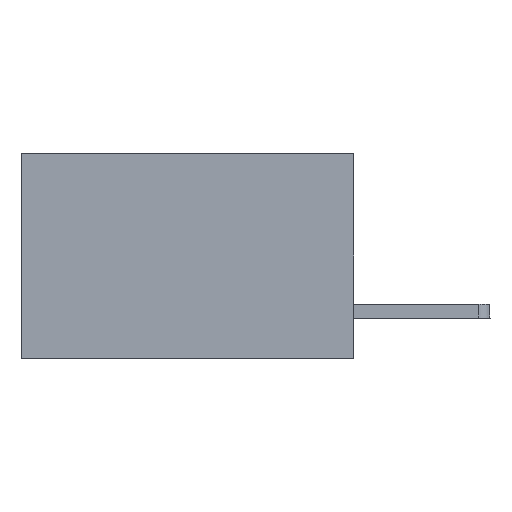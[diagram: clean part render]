
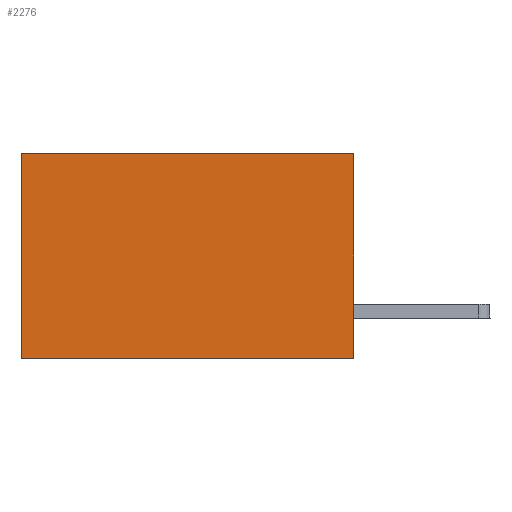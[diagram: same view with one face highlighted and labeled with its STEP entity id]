
A CAD part, left-side view. The second image highlights one B-rep face of the part: STEP entity #2276.
In plain terms, the highlighted planar face has unit normal (-1, 0, 0).
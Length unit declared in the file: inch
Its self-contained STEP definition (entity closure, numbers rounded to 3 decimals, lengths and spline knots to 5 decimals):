
#83 = LINE ( 'NONE', #14897, #2909 ) ;
#582 = EDGE_LOOP ( 'NONE', ( #8738, #12681, #991, #12155 ) ) ;
#651 = VERTEX_POINT ( 'NONE', #6128 ) ;
#991 = ORIENTED_EDGE ( 'NONE', *, *, #5662, .F. ) ;
#1523 = LINE ( 'NONE', #3004, #14735 ) ;
#2205 = DIRECTION ( 'NONE',  ( 0., 0., -1. ) ) ;
#2276 = ADVANCED_FACE ( 'NONE', ( #2409 ), #13121, .F. ) ;
#2409 = FACE_OUTER_BOUND ( 'NONE', #582, .T. ) ;
#2530 = DIRECTION ( 'NONE',  ( 0., 1., 0. ) ) ;
#2909 = VECTOR ( 'NONE', #5752, 39.37008 ) ;
#3004 = CARTESIAN_POINT ( 'NONE',  ( 0.2875, 0., -0.37 ) ) ;
#3277 = EDGE_CURVE ( 'NONE', #11011, #12701, #1523, .T. ) ;
#3392 = CARTESIAN_POINT ( 'NONE',  ( 0.2875, 0., -0.37 ) ) ;
#3790 = VECTOR ( 'NONE', #7036, 39.37008 ) ;
#4533 = EDGE_CURVE ( 'NONE', #651, #12701, #9919, .T. ) ;
#5180 = AXIS2_PLACEMENT_3D ( 'NONE', #12058, #12765, #2205 ) ;
#5662 = EDGE_CURVE ( 'NONE', #13870, #11011, #7246, .T. ) ;
#5752 = DIRECTION ( 'NONE',  ( 0., 1., 0. ) ) ;
#6128 = CARTESIAN_POINT ( 'NONE',  ( 0.2875, 0.6, 0. ) ) ;
#7036 = DIRECTION ( 'NONE',  ( 0., 0., -1. ) ) ;
#7246 = LINE ( 'NONE', #10800, #3790 ) ;
#8738 = ORIENTED_EDGE ( 'NONE', *, *, #4533, .T. ) ;
#9917 = DIRECTION ( 'NONE',  ( 0., 0., -1. ) ) ;
#9919 = LINE ( 'NONE', #12783, #16495 ) ;
#10268 = EDGE_CURVE ( 'NONE', #13870, #651, #83, .T. ) ;
#10800 = CARTESIAN_POINT ( 'NONE',  ( 0.2875, 0., 0. ) ) ;
#10959 = CARTESIAN_POINT ( 'NONE',  ( 0.2875, 0., 0. ) ) ;
#11011 = VERTEX_POINT ( 'NONE', #3392 ) ;
#12058 = CARTESIAN_POINT ( 'NONE',  ( 0.2875, 0., 0. ) ) ;
#12155 = ORIENTED_EDGE ( 'NONE', *, *, #10268, .T. ) ;
#12681 = ORIENTED_EDGE ( 'NONE', *, *, #3277, .F. ) ;
#12701 = VERTEX_POINT ( 'NONE', #15041 ) ;
#12765 = DIRECTION ( 'NONE',  ( 1., 0., 0. ) ) ;
#12783 = CARTESIAN_POINT ( 'NONE',  ( 0.2875, 0.6, 0. ) ) ;
#13121 = PLANE ( 'NONE',  #5180 ) ;
#13870 = VERTEX_POINT ( 'NONE', #10959 ) ;
#14735 = VECTOR ( 'NONE', #2530, 39.37008 ) ;
#14897 = CARTESIAN_POINT ( 'NONE',  ( 0.2875, 0., 0. ) ) ;
#15041 = CARTESIAN_POINT ( 'NONE',  ( 0.2875, 0.6, -0.37 ) ) ;
#16495 = VECTOR ( 'NONE', #9917, 39.37008 ) ;
